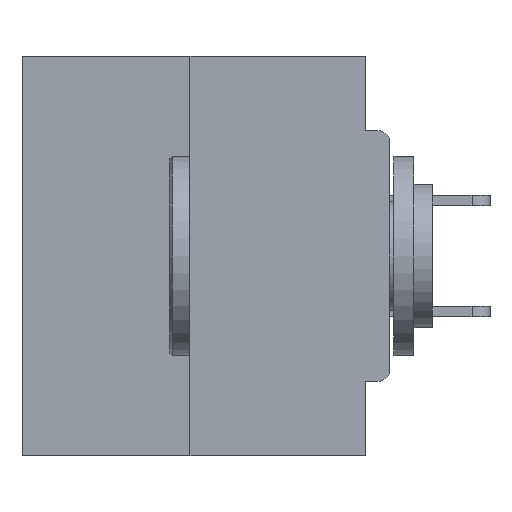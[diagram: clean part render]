
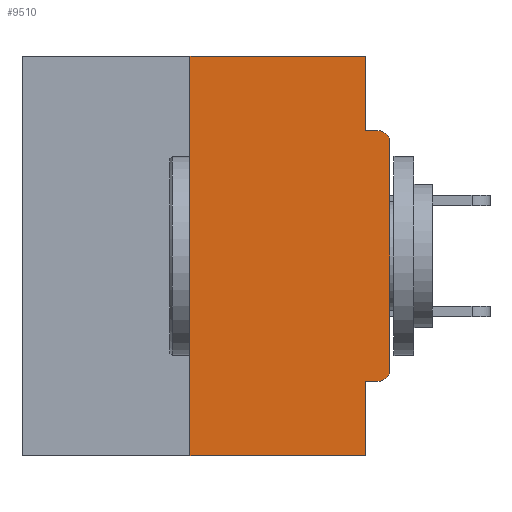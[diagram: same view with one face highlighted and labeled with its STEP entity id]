
A CAD part, left-side view. The second image highlights one B-rep face of the part: STEP entity #9510.
In plain terms, the highlighted planar face has unit normal (-1, 0, 0).
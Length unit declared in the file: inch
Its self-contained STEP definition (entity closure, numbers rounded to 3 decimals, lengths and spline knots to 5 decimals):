
#17 = CARTESIAN_POINT ( 'NONE',  ( 0., 0.25, -0.5 ) ) ;
#279 = DIRECTION ( 'NONE',  ( 0., 0., -1. ) ) ;
#440 = PLANE ( 'NONE',  #24521 ) ;
#573 = LINE ( 'NONE', #32784, #10503 ) ;
#1617 = VERTEX_POINT ( 'NONE', #31973 ) ;
#1720 = ORIENTED_EDGE ( 'NONE', *, *, #22638, .F. ) ;
#2002 = ORIENTED_EDGE ( 'NONE', *, *, #18049, .F. ) ;
#2202 = VECTOR ( 'NONE', #22533, 39.37008 ) ;
#2407 = LINE ( 'NONE', #23104, #30554 ) ;
#2554 = EDGE_CURVE ( 'NONE', #15399, #22537, #16532, .T. ) ;
#2559 = VERTEX_POINT ( 'NONE', #17 ) ;
#2639 = CIRCLE ( 'NONE', #29969, 0.015 ) ;
#2653 = CARTESIAN_POINT ( 'NONE',  ( 0., 0.46, 0. ) ) ;
#2937 = DIRECTION ( 'NONE',  ( -1., 0., 0. ) ) ;
#3298 = CARTESIAN_POINT ( 'NONE',  ( 0., 0.015, -0.1085 ) ) ;
#3328 = ORIENTED_EDGE ( 'NONE', *, *, #2554, .F. ) ;
#4705 = EDGE_CURVE ( 'NONE', #17028, #12317, #33828, .T. ) ;
#5769 = VECTOR ( 'NONE', #27185, 39.37008 ) ;
#5950 = CARTESIAN_POINT ( 'NONE',  ( 0., 0.015, -0.3915 ) ) ;
#6125 = EDGE_CURVE ( 'NONE', #2559, #10258, #17277, .T. ) ;
#6583 = DIRECTION ( 'NONE',  ( 0., 0., 1. ) ) ;
#7410 = CARTESIAN_POINT ( 'NONE',  ( 0., 0.031, 0. ) ) ;
#7471 = LINE ( 'NONE', #7410, #5769 ) ;
#8248 = DIRECTION ( 'NONE',  ( -1., 0., 0. ) ) ;
#8915 = EDGE_CURVE ( 'NONE', #17549, #22327, #573, .T. ) ;
#9510 = ADVANCED_FACE ( 'NONE', ( #32426 ), #440, .F. ) ;
#10258 = VERTEX_POINT ( 'NONE', #33867 ) ;
#10503 = VECTOR ( 'NONE', #33032, 39.37008 ) ;
#10528 = EDGE_CURVE ( 'NONE', #12317, #1617, #32049, .T. ) ;
#10896 = CARTESIAN_POINT ( 'NONE',  ( 0., 0.031, -0.5 ) ) ;
#11120 = VECTOR ( 'NONE', #16743, 39.37008 ) ;
#12317 = VERTEX_POINT ( 'NONE', #12371 ) ;
#12371 = CARTESIAN_POINT ( 'NONE',  ( 0., 0., -0.1085 ) ) ;
#12408 = EDGE_CURVE ( 'NONE', #22327, #10258, #29353, .T. ) ;
#12727 = CARTESIAN_POINT ( 'NONE',  ( 0., 0., -0.3915 ) ) ;
#12943 = VERTEX_POINT ( 'NONE', #16940 ) ;
#12977 = ORIENTED_EDGE ( 'NONE', *, *, #6125, .T. ) ;
#13026 = CARTESIAN_POINT ( 'NONE',  ( 0., 0.031, 0. ) ) ;
#13360 = VECTOR ( 'NONE', #17105, 39.37008 ) ;
#13642 = ORIENTED_EDGE ( 'NONE', *, *, #14729, .F. ) ;
#14442 = DIRECTION ( 'NONE',  ( 0., 0., 1. ) ) ;
#14729 = EDGE_CURVE ( 'NONE', #22537, #12943, #7471, .T. ) ;
#15399 = VERTEX_POINT ( 'NONE', #23097 ) ;
#16532 = LINE ( 'NONE', #2653, #2202 ) ;
#16743 = DIRECTION ( 'NONE',  ( 0., 0., -1. ) ) ;
#16758 = DIRECTION ( 'NONE',  ( 0., 0., -1. ) ) ;
#16912 = DIRECTION ( 'NONE',  ( 0., 0., -1. ) ) ;
#16940 = CARTESIAN_POINT ( 'NONE',  ( 0., 0.031, -0.0935 ) ) ;
#17028 = VERTEX_POINT ( 'NONE', #12727 ) ;
#17105 = DIRECTION ( 'NONE',  ( 0., -1., 0. ) ) ;
#17277 = LINE ( 'NONE', #33792, #13360 ) ;
#17549 = VERTEX_POINT ( 'NONE', #23138 ) ;
#17556 = CARTESIAN_POINT ( 'NONE',  ( 0., 0.031, -0.4065 ) ) ;
#17667 = LINE ( 'NONE', #28858, #25040 ) ;
#18049 = EDGE_CURVE ( 'NONE', #2559, #15399, #17667, .T. ) ;
#20073 = DIRECTION ( 'NONE',  ( 0., -1., 0. ) ) ;
#20664 = ORIENTED_EDGE ( 'NONE', *, *, #4705, .T. ) ;
#22327 = VERTEX_POINT ( 'NONE', #17556 ) ;
#22533 = DIRECTION ( 'NONE',  ( 0., -1., 0. ) ) ;
#22537 = VERTEX_POINT ( 'NONE', #13026 ) ;
#22638 = EDGE_CURVE ( 'NONE', #12943, #1617, #2407, .T. ) ;
#22728 = CARTESIAN_POINT ( 'NONE',  ( 0., 0.46, 0. ) ) ;
#23055 = CARTESIAN_POINT ( 'NONE',  ( 0., 0., 0. ) ) ;
#23097 = CARTESIAN_POINT ( 'NONE',  ( 0., 0.25, 0. ) ) ;
#23104 = CARTESIAN_POINT ( 'NONE',  ( 0., 0., -0.0935 ) ) ;
#23138 = CARTESIAN_POINT ( 'NONE',  ( 0., 0.015, -0.4065 ) ) ;
#24521 = AXIS2_PLACEMENT_3D ( 'NONE', #22728, #30693, #16912 ) ;
#24744 = VECTOR ( 'NONE', #14442, 39.37008 ) ;
#24930 = EDGE_LOOP ( 'NONE', ( #3328, #2002, #12977, #25231, #28264, #27457, #20664, #28079, #1720, #13642 ) ) ;
#25040 = VECTOR ( 'NONE', #6583, 39.37008 ) ;
#25231 = ORIENTED_EDGE ( 'NONE', *, *, #12408, .F. ) ;
#25684 = AXIS2_PLACEMENT_3D ( 'NONE', #3298, #8248, #16758 ) ;
#27185 = DIRECTION ( 'NONE',  ( 0., 0., -1. ) ) ;
#27457 = ORIENTED_EDGE ( 'NONE', *, *, #33493, .T. ) ;
#28079 = ORIENTED_EDGE ( 'NONE', *, *, #10528, .T. ) ;
#28264 = ORIENTED_EDGE ( 'NONE', *, *, #8915, .F. ) ;
#28858 = CARTESIAN_POINT ( 'NONE',  ( 0., 0.25, 0. ) ) ;
#29353 = LINE ( 'NONE', #10896, #11120 ) ;
#29969 = AXIS2_PLACEMENT_3D ( 'NONE', #5950, #2937, #279 ) ;
#30554 = VECTOR ( 'NONE', #20073, 39.37008 ) ;
#30693 = DIRECTION ( 'NONE',  ( 1., 0., 0. ) ) ;
#31973 = CARTESIAN_POINT ( 'NONE',  ( 0., 0.015, -0.0935 ) ) ;
#32049 = CIRCLE ( 'NONE', #25684, 0.015 ) ;
#32426 = FACE_OUTER_BOUND ( 'NONE', #24930, .T. ) ;
#32784 = CARTESIAN_POINT ( 'NONE',  ( 0., 0., -0.4065 ) ) ;
#33032 = DIRECTION ( 'NONE',  ( 0., 1., 0. ) ) ;
#33493 = EDGE_CURVE ( 'NONE', #17549, #17028, #2639, .T. ) ;
#33792 = CARTESIAN_POINT ( 'NONE',  ( 0., 0.46, -0.5 ) ) ;
#33828 = LINE ( 'NONE', #23055, #24744 ) ;
#33867 = CARTESIAN_POINT ( 'NONE',  ( 0., 0.031, -0.5 ) ) ;
